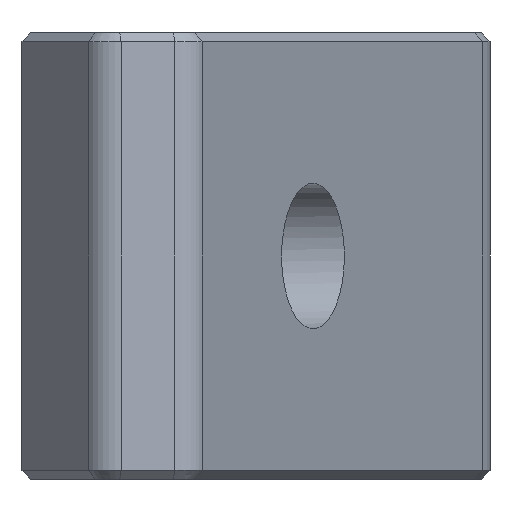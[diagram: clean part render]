
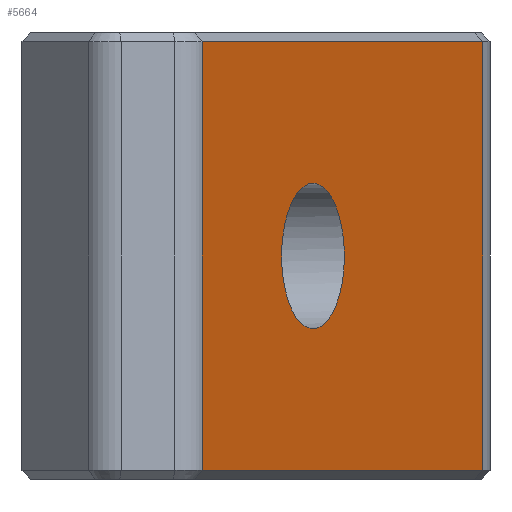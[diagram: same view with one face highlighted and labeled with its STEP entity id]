
A CAD part, left-side view. The second image highlights one B-rep face of the part: STEP entity #5664.
In plain terms, the highlighted planar face has unit normal (-0.396, -0.918, 0).
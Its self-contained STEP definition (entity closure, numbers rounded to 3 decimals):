
#25=ELLIPSE('',#6049,4.437,4.075);
#152=FACE_BOUND('',#801,.T.);
#174=PLANE('',#6048);
#448=FACE_OUTER_BOUND('',#800,.T.);
#800=EDGE_LOOP('',(#4022,#4023,#4024,#4025));
#801=EDGE_LOOP('',(#4026));
#1168=LINE('',#8366,#1768);
#1187=LINE('',#8414,#1787);
#1188=LINE('',#8418,#1788);
#1189=LINE('',#8419,#1789);
#1768=VECTOR('',#6624,10.);
#1787=VECTOR('',#6673,10.);
#1788=VECTOR('',#6678,10.);
#1789=VECTOR('',#6679,10.);
#2543=VERTEX_POINT('',#8356);
#2545=VERTEX_POINT('',#8362);
#2560=VERTEX_POINT('',#8413);
#2561=VERTEX_POINT('',#8417);
#2562=VERTEX_POINT('',#8420);
#3081=EDGE_CURVE('',#2543,#2545,#1168,.T.);
#3105=EDGE_CURVE('',#2545,#2560,#1187,.T.);
#3107=EDGE_CURVE('',#2561,#2543,#1188,.T.);
#3108=EDGE_CURVE('',#2560,#2561,#1189,.T.);
#3109=EDGE_CURVE('',#2562,#2562,#25,.T.);
#4022=ORIENTED_EDGE('',*,*,#3081,.F.);
#4023=ORIENTED_EDGE('',*,*,#3107,.F.);
#4024=ORIENTED_EDGE('',*,*,#3108,.F.);
#4025=ORIENTED_EDGE('',*,*,#3105,.F.);
#4026=ORIENTED_EDGE('',*,*,#3109,.T.);
#5664=ADVANCED_FACE('',(#448,#152),#174,.T.);
#6048=AXIS2_PLACEMENT_3D('',#8416,#6676,#6677);
#6049=AXIS2_PLACEMENT_3D('',#8421,#6680,#6681);
#6624=DIRECTION('',(-0.918,0.396,0.));
#6673=DIRECTION('',(0.,0.,1.));
#6676=DIRECTION('center_axis',(-0.396,-0.918,0.));
#6677=DIRECTION('ref_axis',(-0.918,0.396,0.));
#6678=DIRECTION('',(0.,0.,-1.));
#6679=DIRECTION('',(0.918,-0.396,0.));
#6680=DIRECTION('center_axis',(0.396,0.918,0.));
#6681=DIRECTION('ref_axis',(0.918,-0.396,0.));
#8356=CARTESIAN_POINT('',(256.025,78.191,152.996));
#8362=CARTESIAN_POINT('',(219.587,93.889,152.996));
#8366=CARTESIAN_POINT('',(265.933,73.923,152.996));
#8413=CARTESIAN_POINT('',(219.587,93.889,176.996));
#8414=CARTESIAN_POINT('',(219.587,93.889,164.996));
#8416=CARTESIAN_POINT('Origin',(256.972,77.783,164.996));
#8417=CARTESIAN_POINT('',(256.025,78.191,176.996));
#8418=CARTESIAN_POINT('',(256.025,78.191,164.996));
#8419=CARTESIAN_POINT('',(265.933,73.923,176.996));
#8420=CARTESIAN_POINT('',(229.897,89.448,164.996));
#8421=CARTESIAN_POINT('Origin',(233.972,87.692,164.996));
